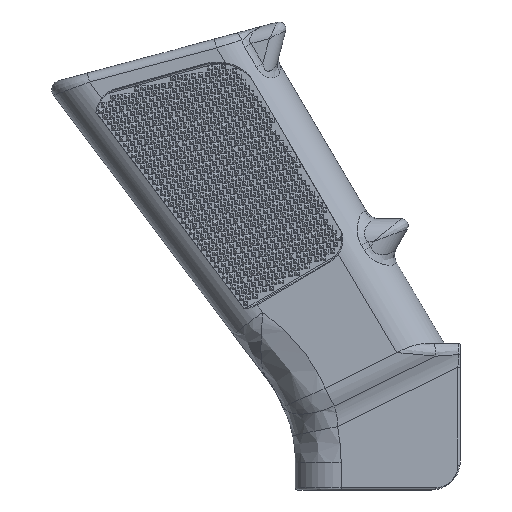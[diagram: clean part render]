
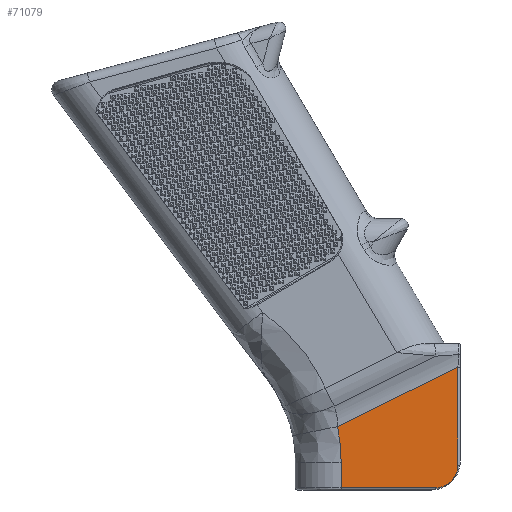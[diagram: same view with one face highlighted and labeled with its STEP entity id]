
A CAD part, front view. The second image highlights one B-rep face of the part: STEP entity #71079.
In plain terms, the highlighted planar face has unit normal (0, -1, 0).
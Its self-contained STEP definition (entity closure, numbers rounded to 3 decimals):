
#344 = CARTESIAN_POINT ( 'NONE',  ( -8., 0., -7.376 ) ) ;
#1865 = FACE_OUTER_BOUND ( 'NONE', #10010, .T. ) ;
#3533 = VECTOR ( 'NONE', #152193, 1000. ) ;
#3818 = CARTESIAN_POINT ( 'NONE',  ( 17.392, 0., -11.625 ) ) ;
#5200 = CARTESIAN_POINT ( 'NONE',  ( -8., 0., 0. ) ) ;
#9566 = EDGE_CURVE ( 'NONE', #45819, #65521, #123398, .T. ) ;
#10010 = EDGE_LOOP ( 'NONE', ( #141982, #65242, #109951, #30751, #139543, #97479 ) ) ;
#11193 = CARTESIAN_POINT ( 'NONE',  ( -0.861, 0., 1.75 ) ) ;
#14636 = CARTESIAN_POINT ( 'NONE',  ( 0., 0., -15.5 ) ) ;
#14785 = CARTESIAN_POINT ( 'NONE',  ( 14.844, 0., -14.961 ) ) ;
#16894 = PLANE ( 'NONE',  #143347 ) ;
#17225 = CARTESIAN_POINT ( 'NONE',  ( 16.484, 0., -13.589 ) ) ;
#24093 = CARTESIAN_POINT ( 'NONE',  ( 14.175, 0., -15.251 ) ) ;
#24917 = CARTESIAN_POINT ( 'NONE',  ( 13.865, 0., -15.345 ) ) ;
#27185 = CARTESIAN_POINT ( 'NONE',  ( -8.262, 0., -4.743 ) ) ;
#29191 = VECTOR ( 'NONE', #116202, 1000. ) ;
#29845 = CARTESIAN_POINT ( 'NONE',  ( 16.337, 0., -13.776 ) ) ;
#30658 = CARTESIAN_POINT ( 'NONE',  ( 17.003, 0., -12.775 ) ) ;
#30751 = ORIENTED_EDGE ( 'NONE', *, *, #94898, .T. ) ;
#34671 = VERTEX_POINT ( 'NONE', #107114 ) ;
#40000 = CARTESIAN_POINT ( 'NONE',  ( 13.467, 0., -15.423 ) ) ;
#40814 = CARTESIAN_POINT ( 'NONE',  ( 12.997, 0., -15.488 ) ) ;
#42470 = CARTESIAN_POINT ( 'NONE',  ( 17.189, 0., -12.325 ) ) ;
#45819 = VERTEX_POINT ( 'NONE', #74589 ) ;
#52603 = CARTESIAN_POINT ( 'NONE',  ( 12.759, 0., -15.5 ) ) ;
#55032 = CARTESIAN_POINT ( 'NONE',  ( 16.579, 0., -13.461 ) ) ;
#55500 = EDGE_CURVE ( 'NONE', #105522, #34671, #125503, .T. ) ;
#56333 = EDGE_CURVE ( 'NONE', #105522, #151366, #79121, .T. ) ;
#56706 = CARTESIAN_POINT ( 'NONE',  ( 17.5, 0., -10.919 ) ) ;
#57255 = CARTESIAN_POINT ( 'NONE',  ( -8., 0., -10.021 ) ) ;
#57524 = CARTESIAN_POINT ( 'NONE',  ( 16.177, 0., -13.952 ) ) ;
#59648 = CARTESIAN_POINT ( 'NONE',  ( 17.5, 0., 0. ) ) ;
#61122 = CARTESIAN_POINT ( 'NONE',  ( 17.5, 0., 10.789 ) ) ;
#65242 = ORIENTED_EDGE ( 'NONE', *, *, #55500, .F. ) ;
#65433 = CARTESIAN_POINT ( 'NONE',  ( -8., 0., -15.5 ) ) ;
#65521 = VERTEX_POINT ( 'NONE', #61122 ) ;
#68513 = EDGE_CURVE ( 'NONE', #65521, #34671, #162268, .T. ) ;
#71079 = ADVANCED_FACE ( 'NONE', ( #1865 ), #16894, .T. ) ;
#74589 = CARTESIAN_POINT ( 'NONE',  ( 17.5, 0., -10.6 ) ) ;
#75327 = CARTESIAN_POINT ( 'NONE',  ( 15.194, 0., -14.758 ) ) ;
#76131 = CARTESIAN_POINT ( 'NONE',  ( 15.055, 0., -14.841 ) ) ;
#79121 = LINE ( 'NONE', #5200, #127092 ) ;
#79422 = CARTESIAN_POINT ( 'NONE',  ( 17.469, 0., -11.234 ) ) ;
#79890 = DIRECTION ( 'NONE',  ( 0., 0., -1. ) ) ;
#80239 = CARTESIAN_POINT ( 'NONE',  ( 15.84, 0., -14.29 ) ) ;
#81057 = CARTESIAN_POINT ( 'NONE',  ( 17.5, 0., -10.6 ) ) ;
#90158 = CARTESIAN_POINT ( 'NONE',  ( -8.782, 0., -2.15 ) ) ;
#91179 = CARTESIAN_POINT ( 'NONE',  ( 14.625, 0., -15.065 ) ) ;
#92004 = CARTESIAN_POINT ( 'NONE',  ( 16.624, 0., -13.397 ) ) ;
#94898 = EDGE_CURVE ( 'NONE', #151366, #116922, #164883, .T. ) ;
#97479 = ORIENTED_EDGE ( 'NONE', *, *, #9566, .T. ) ;
#99907 = DIRECTION ( 'NONE',  ( 0., 0., 1. ) ) ;
#101322 = CARTESIAN_POINT ( 'NONE',  ( 12.6, 0., -15.5 ) ) ;
#103794 = CARTESIAN_POINT ( 'NONE',  ( 13.233, 0., -15.46 ) ) ;
#105081 = CARTESIAN_POINT ( 'NONE',  ( 0., 0., 0. ) ) ;
#105522 = VERTEX_POINT ( 'NONE', #57255 ) ;
#107114 = CARTESIAN_POINT ( 'NONE',  ( -8.782, 0., -2.15 ) ) ;
#109951 = ORIENTED_EDGE ( 'NONE', *, *, #56333, .T. ) ;
#111314 = EDGE_CURVE ( 'NONE', #116922, #45819, #141484, .T. ) ;
#115322 = CARTESIAN_POINT ( 'NONE',  ( -8., 0., -10.021 ) ) ;
#116202 = DIRECTION ( 'NONE',  ( 1., 0., 0. ) ) ;
#116922 = VERTEX_POINT ( 'NONE', #149953 ) ;
#123398 = LINE ( 'NONE', #59648, #148983 ) ;
#125503 =( BOUNDED_CURVE ( )  B_SPLINE_CURVE ( 3, ( #115322, #344, #27185, #90158 ),
 .UNSPECIFIED., .F., .F. ) 
 B_SPLINE_CURVE_WITH_KNOTS ( ( 4, 4 ),
 ( 0., 1. ),
 .UNSPECIFIED. ) 
 CURVE ( )  GEOMETRIC_REPRESENTATION_ITEM ( )  RATIONAL_B_SPLINE_CURVE ( ( 1., 0.997, 0.997, 1. ) ) 
 REPRESENTATION_ITEM ( '' )  );
#127092 = VECTOR ( 'NONE', #159595, 1000. ) ;
#131390 = CARTESIAN_POINT ( 'NONE',  ( 17.374, 0., -11.706 ) ) ;
#132206 = CARTESIAN_POINT ( 'NONE',  ( 16.85, 0., -13.061 ) ) ;
#133547 = DIRECTION ( 'NONE',  ( 0., -1., 0. ) ) ;
#139543 = ORIENTED_EDGE ( 'NONE', *, *, #111314, .T. ) ;
#141484 = B_SPLINE_CURVE_WITH_KNOTS ( 'NONE', 3,
 ( #101322, #52603, #40814, #103794, #154947, #40000, #24917, #24093, #91179, #14785, #76131, #75327, #156570, #146483, #80239, #57524, #29845, #17225, #55032, #92004, #132206, #30658, #42470, #144824, #145640, #131390, #3818, #79422, #56706, #81057 ),
 .UNSPECIFIED., .F., .F.,
 ( 4, 1, 2, 2, 2, 1, 2, 2, 2, 1, 2, 2, 2, 1, 2, 2, 4 ),
 ( 0., 0.063, 0.094, 0.125, 0.25, 0.313, 0.344, 0.375, 0.5, 0.563, 0.594, 0.625, 0.75, 0.812, 0.844, 0.875, 1. ),
 .UNSPECIFIED. ) ;
#141982 = ORIENTED_EDGE ( 'NONE', *, *, #68513, .T. ) ;
#143347 = AXIS2_PLACEMENT_3D ( 'NONE', #105081, #133547, #79890 ) ;
#144824 = CARTESIAN_POINT ( 'NONE',  ( 17.271, 0., -12.097 ) ) ;
#145640 = CARTESIAN_POINT ( 'NONE',  ( 17.335, 0., -11.863 ) ) ;
#146483 = CARTESIAN_POINT ( 'NONE',  ( 15.594, 0., -14.492 ) ) ;
#148983 = VECTOR ( 'NONE', #99907, 1000. ) ;
#149953 = CARTESIAN_POINT ( 'NONE',  ( 12.6, 0., -15.5 ) ) ;
#151366 = VERTEX_POINT ( 'NONE', #65433 ) ;
#152193 = DIRECTION ( 'NONE',  ( -0.897, 0., -0.442 ) ) ;
#154947 = CARTESIAN_POINT ( 'NONE',  ( 13.39, 0., -15.437 ) ) ;
#156570 = CARTESIAN_POINT ( 'NONE',  ( 15.264, 0., -14.713 ) ) ;
#159595 = DIRECTION ( 'NONE',  ( 0., 0., -1. ) ) ;
#162268 = LINE ( 'NONE', #11193, #3533 ) ;
#164883 = LINE ( 'NONE', #14636, #29191 ) ;
